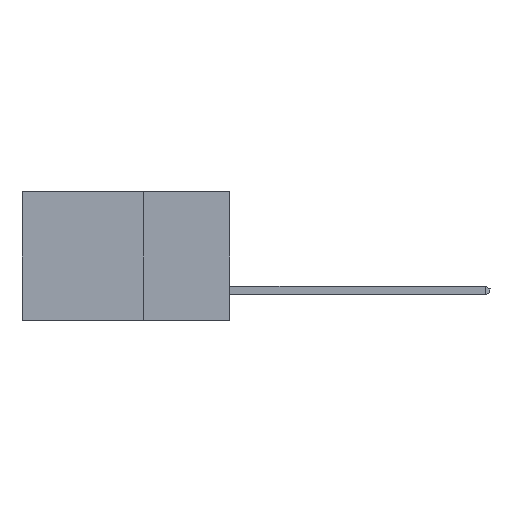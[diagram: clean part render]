
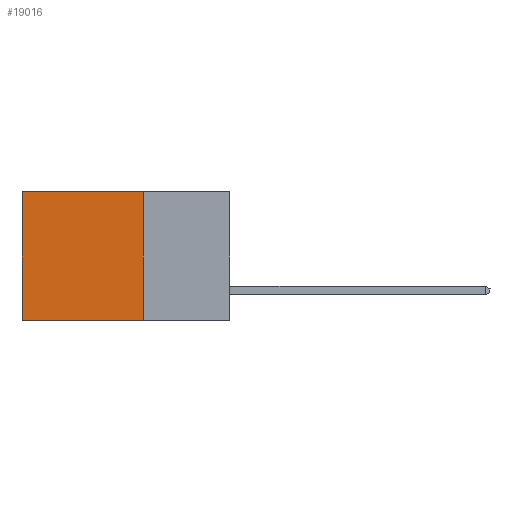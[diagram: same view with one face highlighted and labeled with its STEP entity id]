
A CAD part, left-side view. The second image highlights one B-rep face of the part: STEP entity #19016.
In plain terms, the highlighted planar face has unit normal (-1, 0, 0).
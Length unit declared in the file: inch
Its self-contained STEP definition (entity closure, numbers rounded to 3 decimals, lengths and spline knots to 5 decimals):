
#365 = EDGE_CURVE ( 'NONE', #7929, #6282, #7875, .T. ) ;
#1095 = DIRECTION ( 'NONE',  ( 0., 0., -1. ) ) ;
#1665 = CARTESIAN_POINT ( 'NONE',  ( 0.2615, 0.25, -0.37 ) ) ;
#1726 = VECTOR ( 'NONE', #1095, 39.37008 ) ;
#2970 = EDGE_CURVE ( 'NONE', #4044, #8526, #4210, .T. ) ;
#3002 = ORIENTED_EDGE ( 'NONE', *, *, #2970, .T. ) ;
#3263 = EDGE_LOOP ( 'NONE', ( #3002, #15252, #20494, #3989 ) ) ;
#3309 = DIRECTION ( 'NONE',  ( 0., 0., -1. ) ) ;
#3513 = CARTESIAN_POINT ( 'NONE',  ( 0.2615, 0.25, 0. ) ) ;
#3614 = DIRECTION ( 'NONE',  ( 0., 1., 0. ) ) ;
#3989 = ORIENTED_EDGE ( 'NONE', *, *, #13130, .T. ) ;
#4044 = VERTEX_POINT ( 'NONE', #7781 ) ;
#4210 = LINE ( 'NONE', #4519, #1726 ) ;
#4519 = CARTESIAN_POINT ( 'NONE',  ( 0.2615, 0.6, -0.37 ) ) ;
#4908 = CARTESIAN_POINT ( 'NONE',  ( 0.2615, 0.25, -0.37 ) ) ;
#5013 = DIRECTION ( 'NONE',  ( 0., 1., 0. ) ) ;
#5355 = EDGE_CURVE ( 'NONE', #6282, #8526, #14852, .T. ) ;
#5886 = VECTOR ( 'NONE', #3614, 39.37008 ) ;
#6126 = CARTESIAN_POINT ( 'NONE',  ( 0.2615, 0.6, -0.37 ) ) ;
#6282 = VERTEX_POINT ( 'NONE', #20254 ) ;
#6483 = FACE_OUTER_BOUND ( 'NONE', #3263, .T. ) ;
#7781 = CARTESIAN_POINT ( 'NONE',  ( 0.2615, 0.6, 0. ) ) ;
#7875 = LINE ( 'NONE', #1665, #18067 ) ;
#7929 = VERTEX_POINT ( 'NONE', #10260 ) ;
#8526 = VERTEX_POINT ( 'NONE', #6126 ) ;
#10260 = CARTESIAN_POINT ( 'NONE',  ( 0.2615, 0.25, 0. ) ) ;
#11255 = AXIS2_PLACEMENT_3D ( 'NONE', #4908, #11426, #3309 ) ;
#11426 = DIRECTION ( 'NONE',  ( 1., 0., 0. ) ) ;
#11521 = CARTESIAN_POINT ( 'NONE',  ( 0.2615, 0.25, -0.37 ) ) ;
#13032 = PLANE ( 'NONE',  #11255 ) ;
#13130 = EDGE_CURVE ( 'NONE', #7929, #4044, #18167, .T. ) ;
#14416 = DIRECTION ( 'NONE',  ( 0., 0., -1. ) ) ;
#14852 = LINE ( 'NONE', #11521, #5886 ) ;
#15252 = ORIENTED_EDGE ( 'NONE', *, *, #5355, .F. ) ;
#17655 = VECTOR ( 'NONE', #5013, 39.37008 ) ;
#18067 = VECTOR ( 'NONE', #14416, 39.37008 ) ;
#18167 = LINE ( 'NONE', #3513, #17655 ) ;
#19016 = ADVANCED_FACE ( 'NONE', ( #6483 ), #13032, .F. ) ;
#20254 = CARTESIAN_POINT ( 'NONE',  ( 0.2615, 0.25, -0.37 ) ) ;
#20494 = ORIENTED_EDGE ( 'NONE', *, *, #365, .F. ) ;
